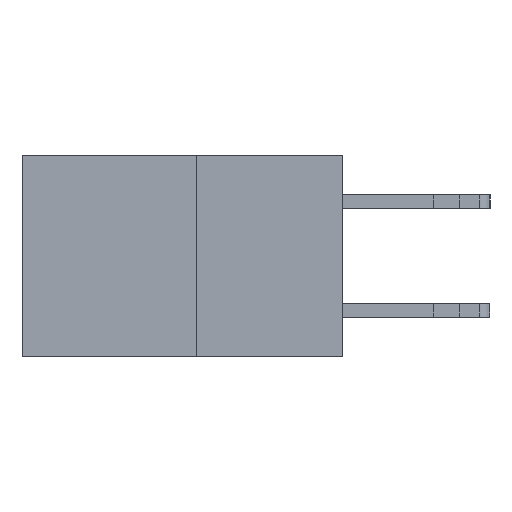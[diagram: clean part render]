
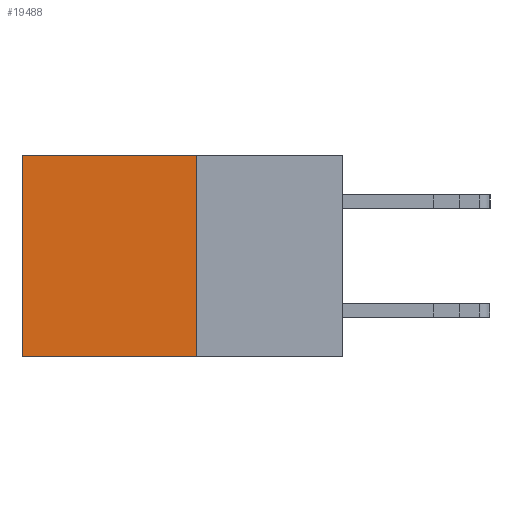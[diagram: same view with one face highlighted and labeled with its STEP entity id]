
A CAD part, left-side view. The second image highlights one B-rep face of the part: STEP entity #19488.
In plain terms, the highlighted planar face has unit normal (-1, 0, 0).
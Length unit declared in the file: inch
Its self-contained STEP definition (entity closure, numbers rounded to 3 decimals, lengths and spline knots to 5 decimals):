
#2059 = CARTESIAN_POINT ( 'NONE',  ( 0.277, 0.27, -0.37 ) ) ;
#2103 = DIRECTION ( 'NONE',  ( 0., 1., 0. ) ) ;
#2553 = LINE ( 'NONE', #9512, #25595 ) ;
#3083 = DIRECTION ( 'NONE',  ( 0., 0., -1. ) ) ;
#4087 = VECTOR ( 'NONE', #28736, 39.37008 ) ;
#4309 = LINE ( 'NONE', #15422, #21406 ) ;
#5339 = EDGE_CURVE ( 'NONE', #19224, #16244, #2553, .T. ) ;
#5683 = VECTOR ( 'NONE', #15368, 39.37008 ) ;
#5963 = CARTESIAN_POINT ( 'NONE',  ( 0.277, 0.27, -0.37 ) ) ;
#7761 = ORIENTED_EDGE ( 'NONE', *, *, #15060, .F. ) ;
#8727 = CARTESIAN_POINT ( 'NONE',  ( 0.277, 0.59, -0.37 ) ) ;
#9512 = CARTESIAN_POINT ( 'NONE',  ( 0.277, 0.27, -0.37 ) ) ;
#9607 = CARTESIAN_POINT ( 'NONE',  ( 0.277, 0.27, -0.37 ) ) ;
#10006 = LINE ( 'NONE', #26500, #4087 ) ;
#11296 = ORIENTED_EDGE ( 'NONE', *, *, #5339, .F. ) ;
#11604 = LINE ( 'NONE', #2059, #5683 ) ;
#11922 = EDGE_CURVE ( 'NONE', #18067, #26608, #10006, .T. ) ;
#12466 = DIRECTION ( 'NONE',  ( 0., 0., -1. ) ) ;
#12844 = ORIENTED_EDGE ( 'NONE', *, *, #11922, .T. ) ;
#13940 = EDGE_CURVE ( 'NONE', #19224, #18067, #4309, .T. ) ;
#14161 = PLANE ( 'NONE',  #18061 ) ;
#15060 = EDGE_CURVE ( 'NONE', #16244, #26608, #11604, .T. ) ;
#15368 = DIRECTION ( 'NONE',  ( 0., 1., 0. ) ) ;
#15422 = CARTESIAN_POINT ( 'NONE',  ( 0.277, 0.27, 0. ) ) ;
#16244 = VERTEX_POINT ( 'NONE', #5963 ) ;
#16401 = DIRECTION ( 'NONE',  ( 1., 0., 0. ) ) ;
#18061 = AXIS2_PLACEMENT_3D ( 'NONE', #9607, #16401, #3083 ) ;
#18067 = VERTEX_POINT ( 'NONE', #18710 ) ;
#18710 = CARTESIAN_POINT ( 'NONE',  ( 0.277, 0.59, 0. ) ) ;
#19224 = VERTEX_POINT ( 'NONE', #24575 ) ;
#19488 = ADVANCED_FACE ( 'NONE', ( #25999 ), #14161, .F. ) ;
#19752 = EDGE_LOOP ( 'NONE', ( #12844, #7761, #11296, #23499 ) ) ;
#21406 = VECTOR ( 'NONE', #2103, 39.37008 ) ;
#23499 = ORIENTED_EDGE ( 'NONE', *, *, #13940, .T. ) ;
#24575 = CARTESIAN_POINT ( 'NONE',  ( 0.277, 0.27, 0. ) ) ;
#25595 = VECTOR ( 'NONE', #12466, 39.37008 ) ;
#25999 = FACE_OUTER_BOUND ( 'NONE', #19752, .T. ) ;
#26500 = CARTESIAN_POINT ( 'NONE',  ( 0.277, 0.59, -0.37 ) ) ;
#26608 = VERTEX_POINT ( 'NONE', #8727 ) ;
#28736 = DIRECTION ( 'NONE',  ( 0., 0., -1. ) ) ;
